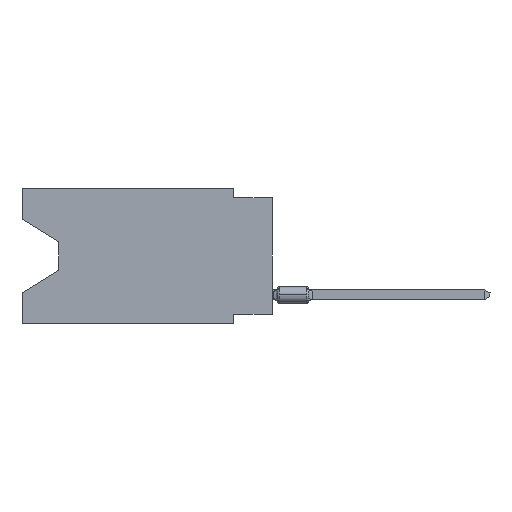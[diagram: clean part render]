
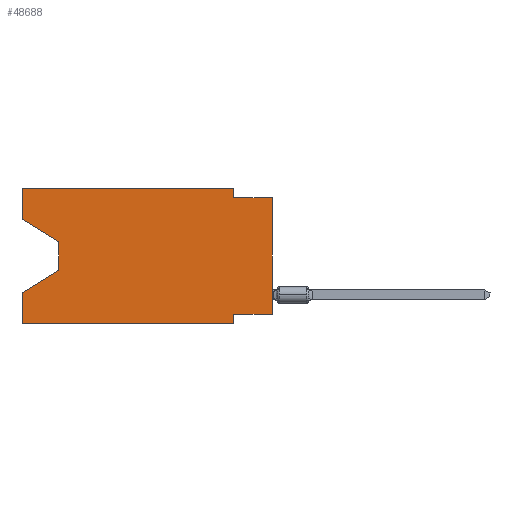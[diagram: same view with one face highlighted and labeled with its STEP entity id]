
A CAD part, left-side view. The second image highlights one B-rep face of the part: STEP entity #48688.
In plain terms, the highlighted planar face has unit normal (-1, 0, 0).
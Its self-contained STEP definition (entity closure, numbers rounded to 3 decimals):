
#224 = CARTESIAN_POINT ( 'NONE',  ( 0., 2.54, -8.255 ) ) ;
#574 = CARTESIAN_POINT ( 'NONE',  ( 0., 16.383, 0. ) ) ;
#1595 = CARTESIAN_POINT ( 'NONE',  ( 0., 2.54, 0. ) ) ;
#1728 = VECTOR ( 'NONE', #96326, 1000. ) ;
#2803 = DIRECTION ( 'NONE',  ( 0., 0., 1. ) ) ;
#3260 = LINE ( 'NONE', #11581, #67661 ) ;
#3594 = ORIENTED_EDGE ( 'NONE', *, *, #77671, .F. ) ;
#6770 = VERTEX_POINT ( 'NONE', #224 ) ;
#6926 = DIRECTION ( 'NONE',  ( 0., 0., -1. ) ) ;
#7778 = VECTOR ( 'NONE', #55639, 1000. ) ;
#8013 = LINE ( 'NONE', #40718, #14534 ) ;
#8315 = EDGE_CURVE ( 'NONE', #6770, #17084, #98801, .T. ) ;
#8489 = EDGE_CURVE ( 'NONE', #63225, #56200, #40568, .T. ) ;
#9733 = EDGE_CURVE ( 'NONE', #82638, #39711, #8013, .T. ) ;
#10044 = DIRECTION ( 'NONE',  ( 0., 0.855, -0.519 ) ) ;
#11581 = CARTESIAN_POINT ( 'NONE',  ( 0., 16.383, -2.038 ) ) ;
#12128 = EDGE_CURVE ( 'NONE', #89836, #43054, #26643, .T. ) ;
#13049 = LINE ( 'NONE', #69131, #16567 ) ;
#13180 = ORIENTED_EDGE ( 'NONE', *, *, #9733, .T. ) ;
#14534 = VECTOR ( 'NONE', #95220, 1000. ) ;
#16567 = VECTOR ( 'NONE', #44724, 1000. ) ;
#17084 = VERTEX_POINT ( 'NONE', #64085 ) ;
#18883 = EDGE_CURVE ( 'NONE', #45995, #63225, #57070, .T. ) ;
#19653 = VERTEX_POINT ( 'NONE', #101882 ) ;
#19737 = CARTESIAN_POINT ( 'NONE',  ( 0., 16.383, 0. ) ) ;
#20334 = ORIENTED_EDGE ( 'NONE', *, *, #31769, .T. ) ;
#20389 = CARTESIAN_POINT ( 'NONE',  ( 0., 0., -8.255 ) ) ;
#21625 = CARTESIAN_POINT ( 'NONE',  ( 0., 13.97, -3.505 ) ) ;
#22144 = CARTESIAN_POINT ( 'NONE',  ( 0., 13.97, -5.385 ) ) ;
#23001 = VERTEX_POINT ( 'NONE', #77506 ) ;
#23151 = ORIENTED_EDGE ( 'NONE', *, *, #18883, .F. ) ;
#25382 = CARTESIAN_POINT ( 'NONE',  ( 0., 16.383, 0. ) ) ;
#26643 = LINE ( 'NONE', #73925, #102702 ) ;
#30950 = LINE ( 'NONE', #21625, #32546 ) ;
#31117 = AXIS2_PLACEMENT_3D ( 'NONE', #69781, #46405, #6926 ) ;
#31233 = LINE ( 'NONE', #101844, #88627 ) ;
#31769 = EDGE_CURVE ( 'NONE', #23001, #17084, #55344, .T. ) ;
#32546 = VECTOR ( 'NONE', #78709, 1000. ) ;
#32934 = CARTESIAN_POINT ( 'NONE',  ( 0., 16.383, 0. ) ) ;
#38220 = CARTESIAN_POINT ( 'NONE',  ( 0., 0., -0.635 ) ) ;
#38343 = EDGE_LOOP ( 'NONE', ( #41270, #67819, #66394, #3594, #20334, #83644, #68901, #13180, #101554, #40064, #89748, #23151 ) ) ;
#39711 = VERTEX_POINT ( 'NONE', #38220 ) ;
#40064 = ORIENTED_EDGE ( 'NONE', *, *, #56080, .F. ) ;
#40568 = LINE ( 'NONE', #574, #7778 ) ;
#40718 = CARTESIAN_POINT ( 'NONE',  ( 0., 0., 0. ) ) ;
#41270 = ORIENTED_EDGE ( 'NONE', *, *, #75745, .T. ) ;
#41307 = CARTESIAN_POINT ( 'NONE',  ( 0., 16.383, -8.89 ) ) ;
#41391 = VECTOR ( 'NONE', #2803, 1000. ) ;
#42184 = CARTESIAN_POINT ( 'NONE',  ( 0., 0., -8.255 ) ) ;
#43054 = VERTEX_POINT ( 'NONE', #99517 ) ;
#44724 = DIRECTION ( 'NONE',  ( 0., -1., 0. ) ) ;
#45995 = VERTEX_POINT ( 'NONE', #63068 ) ;
#46405 = DIRECTION ( 'NONE',  ( 1., 0., 0. ) ) ;
#48688 = ADVANCED_FACE ( 'NONE', ( #62532 ), #68264, .F. ) ;
#49522 = DIRECTION ( 'NONE',  ( 0., -0.855, -0.519 ) ) ;
#50806 = EDGE_CURVE ( 'NONE', #67404, #39711, #13049, .T. ) ;
#55019 = DIRECTION ( 'NONE',  ( 0., 0., 1. ) ) ;
#55344 = LINE ( 'NONE', #41307, #1728 ) ;
#55639 = DIRECTION ( 'NONE',  ( 0., -1., 0. ) ) ;
#56080 = EDGE_CURVE ( 'NONE', #56200, #67404, #31233, .T. ) ;
#56200 = VERTEX_POINT ( 'NONE', #1595 ) ;
#57070 = LINE ( 'NONE', #25382, #87452 ) ;
#59371 = DIRECTION ( 'NONE',  ( 0., 0., -1. ) ) ;
#60399 = LINE ( 'NONE', #20389, #102534 ) ;
#60915 = DIRECTION ( 'NONE',  ( 0., 1., 0. ) ) ;
#62532 = FACE_OUTER_BOUND ( 'NONE', #38343, .T. ) ;
#63068 = CARTESIAN_POINT ( 'NONE',  ( 0., 16.383, -2.038 ) ) ;
#63225 = VERTEX_POINT ( 'NONE', #19737 ) ;
#64085 = CARTESIAN_POINT ( 'NONE',  ( 0., 2.54, -8.89 ) ) ;
#66394 = ORIENTED_EDGE ( 'NONE', *, *, #12128, .T. ) ;
#67148 = CARTESIAN_POINT ( 'NONE',  ( 0., 2.54, -8.89 ) ) ;
#67404 = VERTEX_POINT ( 'NONE', #86747 ) ;
#67661 = VECTOR ( 'NONE', #49522, 1000. ) ;
#67819 = ORIENTED_EDGE ( 'NONE', *, *, #70381, .T. ) ;
#68264 = PLANE ( 'NONE',  #31117 ) ;
#68901 = ORIENTED_EDGE ( 'NONE', *, *, #75904, .F. ) ;
#69131 = CARTESIAN_POINT ( 'NONE',  ( 0., 0., -0.635 ) ) ;
#69781 = CARTESIAN_POINT ( 'NONE',  ( 0., 16.383, 0. ) ) ;
#70381 = EDGE_CURVE ( 'NONE', #19653, #89836, #30950, .T. ) ;
#73925 = CARTESIAN_POINT ( 'NONE',  ( 0., 13.97, -5.385 ) ) ;
#75745 = EDGE_CURVE ( 'NONE', #45995, #19653, #3260, .T. ) ;
#75904 = EDGE_CURVE ( 'NONE', #82638, #6770, #60399, .T. ) ;
#77506 = CARTESIAN_POINT ( 'NONE',  ( 0., 16.383, -8.89 ) ) ;
#77671 = EDGE_CURVE ( 'NONE', #23001, #43054, #98322, .T. ) ;
#78709 = DIRECTION ( 'NONE',  ( 0., 0., -1. ) ) ;
#79511 = DIRECTION ( 'NONE',  ( 0., 0., -1. ) ) ;
#82638 = VERTEX_POINT ( 'NONE', #42184 ) ;
#83644 = ORIENTED_EDGE ( 'NONE', *, *, #8315, .F. ) ;
#86747 = CARTESIAN_POINT ( 'NONE',  ( 0., 2.54, -0.635 ) ) ;
#87452 = VECTOR ( 'NONE', #55019, 1000. ) ;
#88627 = VECTOR ( 'NONE', #79511, 1000. ) ;
#89748 = ORIENTED_EDGE ( 'NONE', *, *, #8489, .F. ) ;
#89836 = VERTEX_POINT ( 'NONE', #22144 ) ;
#95220 = DIRECTION ( 'NONE',  ( 0., 0., 1. ) ) ;
#96326 = DIRECTION ( 'NONE',  ( 0., -1., 0. ) ) ;
#98322 = LINE ( 'NONE', #32934, #41391 ) ;
#98801 = LINE ( 'NONE', #67148, #98927 ) ;
#98927 = VECTOR ( 'NONE', #59371, 1000. ) ;
#99517 = CARTESIAN_POINT ( 'NONE',  ( 0., 16.383, -6.852 ) ) ;
#101554 = ORIENTED_EDGE ( 'NONE', *, *, #50806, .F. ) ;
#101844 = CARTESIAN_POINT ( 'NONE',  ( 0., 2.54, 0. ) ) ;
#101882 = CARTESIAN_POINT ( 'NONE',  ( 0., 13.97, -3.505 ) ) ;
#102534 = VECTOR ( 'NONE', #60915, 1000. ) ;
#102702 = VECTOR ( 'NONE', #10044, 1000. ) ;
